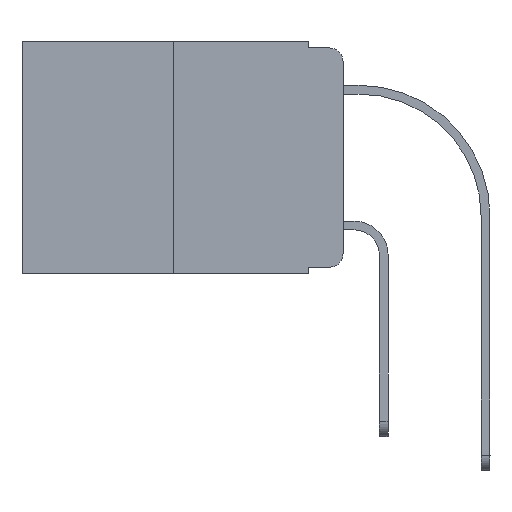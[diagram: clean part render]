
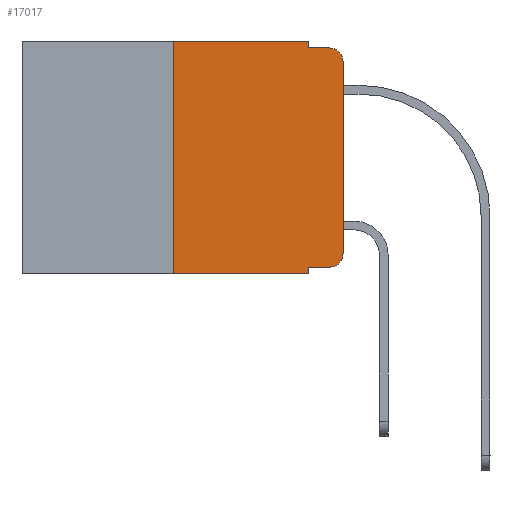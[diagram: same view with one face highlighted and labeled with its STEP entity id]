
A CAD part, left-side view. The second image highlights one B-rep face of the part: STEP entity #17017.
In plain terms, the highlighted planar face has unit normal (-1, 0, 0).
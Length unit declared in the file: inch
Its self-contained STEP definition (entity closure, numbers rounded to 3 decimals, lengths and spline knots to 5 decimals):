
#10 = CARTESIAN_POINT ( 'NONE',  ( 0., 0.051, 0. ) ) ;
#67 = VERTEX_POINT ( 'NONE', #12888 ) ;
#115 = LINE ( 'NONE', #7286, #14983 ) ;
#408 = ORIENTED_EDGE ( 'NONE', *, *, #13180, .F. ) ;
#1573 = LINE ( 'NONE', #12603, #2325 ) ;
#1588 = DIRECTION ( 'NONE',  ( 0., -1., 0. ) ) ;
#1746 = DIRECTION ( 'NONE',  ( 0., -1., 0. ) ) ;
#1876 = CARTESIAN_POINT ( 'NONE',  ( 0., 0.051, 0. ) ) ;
#2243 = CARTESIAN_POINT ( 'NONE',  ( 0., 0.473, 0. ) ) ;
#2267 = EDGE_CURVE ( 'NONE', #17827, #67, #12356, .T. ) ;
#2325 = VECTOR ( 'NONE', #1746, 39.37008 ) ;
#2618 = VERTEX_POINT ( 'NONE', #1876 ) ;
#2796 = EDGE_CURVE ( 'NONE', #17216, #16473, #7098, .T. ) ;
#3106 = ORIENTED_EDGE ( 'NONE', *, *, #15437, .T. ) ;
#3166 = VERTEX_POINT ( 'NONE', #13614 ) ;
#3259 = EDGE_CURVE ( 'NONE', #67, #7810, #13943, .T. ) ;
#3264 = VERTEX_POINT ( 'NONE', #11210 ) ;
#3369 = VECTOR ( 'NONE', #8142, 39.37008 ) ;
#3456 = CARTESIAN_POINT ( 'NONE',  ( 0., 0.25, 0. ) ) ;
#3531 = CARTESIAN_POINT ( 'NONE',  ( 0., 0.051, -0.343 ) ) ;
#3977 = VECTOR ( 'NONE', #14730, 39.37008 ) ;
#4097 = CARTESIAN_POINT ( 'NONE',  ( 0., 0.02, -0.313 ) ) ;
#4128 = CARTESIAN_POINT ( 'NONE',  ( 0., 0.02, -0.01 ) ) ;
#4181 = EDGE_CURVE ( 'NONE', #2618, #3264, #9532, .T. ) ;
#4454 = CARTESIAN_POINT ( 'NONE',  ( 0., 0.051, -0.01 ) ) ;
#4517 = VERTEX_POINT ( 'NONE', #9477 ) ;
#4723 = LINE ( 'NONE', #11911, #3977 ) ;
#5348 = DIRECTION ( 'NONE',  ( 0., 0., -1. ) ) ;
#5516 = CARTESIAN_POINT ( 'NONE',  ( 0., 0.02, -0.03 ) ) ;
#5845 = LINE ( 'NONE', #4454, #11184 ) ;
#5870 = CARTESIAN_POINT ( 'NONE',  ( 0., 0., -0.313 ) ) ;
#5946 = AXIS2_PLACEMENT_3D ( 'NONE', #2243, #13457, #13884 ) ;
#5992 = ORIENTED_EDGE ( 'NONE', *, *, #2267, .T. ) ;
#6800 = EDGE_CURVE ( 'NONE', #3264, #7810, #5845, .T. ) ;
#7020 = LINE ( 'NONE', #15267, #15634 ) ;
#7098 = LINE ( 'NONE', #10, #11235 ) ;
#7203 = CIRCLE ( 'NONE', #10441, 0.02 ) ;
#7286 = CARTESIAN_POINT ( 'NONE',  ( 0., 0.051, -0.333 ) ) ;
#7706 = DIRECTION ( 'NONE',  ( 0., 0., 1. ) ) ;
#7781 = EDGE_CURVE ( 'NONE', #4517, #16473, #1573, .T. ) ;
#7810 = VERTEX_POINT ( 'NONE', #4128 ) ;
#8142 = DIRECTION ( 'NONE',  ( 0., 0., -1. ) ) ;
#8215 = ORIENTED_EDGE ( 'NONE', *, *, #2796, .F. ) ;
#8626 = DIRECTION ( 'NONE',  ( -1., 0., 0. ) ) ;
#8708 = DIRECTION ( 'NONE',  ( 0., -1., 0. ) ) ;
#9077 = CARTESIAN_POINT ( 'NONE',  ( 0., 0., 0. ) ) ;
#9477 = CARTESIAN_POINT ( 'NONE',  ( 0., 0.25, -0.343 ) ) ;
#9532 = LINE ( 'NONE', #15112, #3369 ) ;
#9724 = DIRECTION ( 'NONE',  ( 0., 0., -1. ) ) ;
#10128 = CARTESIAN_POINT ( 'NONE',  ( 0., 0.051, -0.333 ) ) ;
#10441 = AXIS2_PLACEMENT_3D ( 'NONE', #4097, #8626, #9724 ) ;
#10714 = EDGE_LOOP ( 'NONE', ( #5992, #15964, #15720, #12400, #12023, #408, #11883, #8215, #3106, #11944 ) ) ;
#10974 = EDGE_CURVE ( 'NONE', #3166, #17827, #7203, .T. ) ;
#11184 = VECTOR ( 'NONE', #8708, 39.37008 ) ;
#11210 = CARTESIAN_POINT ( 'NONE',  ( 0., 0.051, -0.01 ) ) ;
#11235 = VECTOR ( 'NONE', #5348, 39.37008 ) ;
#11572 = VECTOR ( 'NONE', #7706, 39.37008 ) ;
#11883 = ORIENTED_EDGE ( 'NONE', *, *, #7781, .T. ) ;
#11911 = CARTESIAN_POINT ( 'NONE',  ( 0., 0.473, 0. ) ) ;
#11944 = ORIENTED_EDGE ( 'NONE', *, *, #10974, .T. ) ;
#12023 = ORIENTED_EDGE ( 'NONE', *, *, #13932, .F. ) ;
#12356 = LINE ( 'NONE', #9077, #11572 ) ;
#12400 = ORIENTED_EDGE ( 'NONE', *, *, #4181, .F. ) ;
#12401 = DIRECTION ( 'NONE',  ( 0., 0., -1. ) ) ;
#12603 = CARTESIAN_POINT ( 'NONE',  ( 0., 0.473, -0.343 ) ) ;
#12623 = DIRECTION ( 'NONE',  ( 0., 0., 1. ) ) ;
#12888 = CARTESIAN_POINT ( 'NONE',  ( 0., 0., -0.03 ) ) ;
#13180 = EDGE_CURVE ( 'NONE', #4517, #14800, #7020, .T. ) ;
#13457 = DIRECTION ( 'NONE',  ( 1., 0., 0. ) ) ;
#13614 = CARTESIAN_POINT ( 'NONE',  ( 0., 0.02, -0.333 ) ) ;
#13884 = DIRECTION ( 'NONE',  ( 0., 0., -1. ) ) ;
#13932 = EDGE_CURVE ( 'NONE', #14800, #2618, #4723, .T. ) ;
#13943 = CIRCLE ( 'NONE', #16282, 0.02 ) ;
#14730 = DIRECTION ( 'NONE',  ( 0., -1., 0. ) ) ;
#14800 = VERTEX_POINT ( 'NONE', #3456 ) ;
#14983 = VECTOR ( 'NONE', #1588, 39.37008 ) ;
#15112 = CARTESIAN_POINT ( 'NONE',  ( 0., 0.051, 0. ) ) ;
#15267 = CARTESIAN_POINT ( 'NONE',  ( 0., 0.25, 0. ) ) ;
#15437 = EDGE_CURVE ( 'NONE', #17216, #3166, #115, .T. ) ;
#15634 = VECTOR ( 'NONE', #12623, 39.37008 ) ;
#15720 = ORIENTED_EDGE ( 'NONE', *, *, #6800, .F. ) ;
#15964 = ORIENTED_EDGE ( 'NONE', *, *, #3259, .T. ) ;
#16191 = PLANE ( 'NONE',  #5946 ) ;
#16282 = AXIS2_PLACEMENT_3D ( 'NONE', #5516, #16692, #12401 ) ;
#16473 = VERTEX_POINT ( 'NONE', #3531 ) ;
#16692 = DIRECTION ( 'NONE',  ( -1., 0., 0. ) ) ;
#17017 = ADVANCED_FACE ( 'NONE', ( #17563 ), #16191, .F. ) ;
#17216 = VERTEX_POINT ( 'NONE', #10128 ) ;
#17563 = FACE_OUTER_BOUND ( 'NONE', #10714, .T. ) ;
#17827 = VERTEX_POINT ( 'NONE', #5870 ) ;
